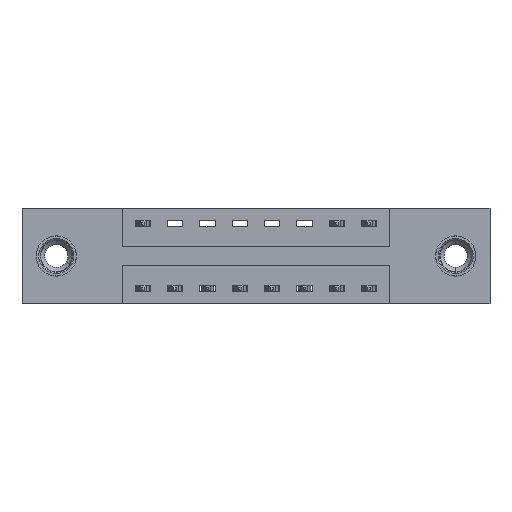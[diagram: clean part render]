
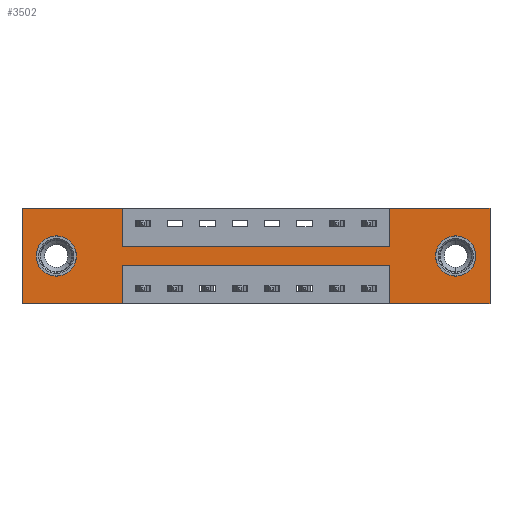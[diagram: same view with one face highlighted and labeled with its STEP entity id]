
A CAD part, front view. The second image highlights one B-rep face of the part: STEP entity #3502.
In plain terms, the highlighted planar face has unit normal (0, -1, 0).
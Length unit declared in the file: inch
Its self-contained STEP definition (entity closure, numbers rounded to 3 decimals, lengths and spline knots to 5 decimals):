
#41 = CARTESIAN_POINT ( 'NONE',  ( 1.6775, 0., -0.185 ) ) ;
#105 = EDGE_CURVE ( 'NONE', #7333, #7266, #4908, .T. ) ;
#182 = LINE ( 'NONE', #8003, #8861 ) ;
#215 = VERTEX_POINT ( 'NONE', #946 ) ;
#295 = LINE ( 'NONE', #981, #8973 ) ;
#345 = DIRECTION ( 'NONE',  ( 0., 0., -1. ) ) ;
#397 = VERTEX_POINT ( 'NONE', #3533 ) ;
#488 = EDGE_CURVE ( 'NONE', #3770, #2480, #9300, .T. ) ;
#666 = VERTEX_POINT ( 'NONE', #4790 ) ;
#691 = LINE ( 'NONE', #5946, #9341 ) ;
#784 = DIRECTION ( 'NONE',  ( -1., 0., 0. ) ) ;
#863 = DIRECTION ( 'NONE',  ( 0., -1., 0. ) ) ;
#910 = DIRECTION ( 'NONE',  ( 0., 0., -1. ) ) ;
#946 = CARTESIAN_POINT ( 'NONE',  ( 0.3875, 0., -0.22 ) ) ;
#981 = CARTESIAN_POINT ( 'NONE',  ( 0., 0., 0. ) ) ;
#1064 = EDGE_CURVE ( 'NONE', #2480, #215, #182, .T. ) ;
#1230 = CARTESIAN_POINT ( 'NONE',  ( 0., 0., -0.37 ) ) ;
#1232 = EDGE_CURVE ( 'NONE', #6895, #3770, #10660, .T. ) ;
#1427 = VERTEX_POINT ( 'NONE', #7745 ) ;
#1442 = EDGE_CURVE ( 'NONE', #7266, #7333, #2202, .T. ) ;
#1566 = AXIS2_PLACEMENT_3D ( 'NONE', #41, #5985, #910 ) ;
#1596 = DIRECTION ( 'NONE',  ( 0., 0., 1. ) ) ;
#1646 = AXIS2_PLACEMENT_3D ( 'NONE', #5944, #863, #6769 ) ;
#1651 = CARTESIAN_POINT ( 'NONE',  ( 1.6775, 0., -0.185 ) ) ;
#1705 = LINE ( 'NONE', #7407, #5918 ) ;
#1753 = CARTESIAN_POINT ( 'NONE',  ( 1.81, 0., 0. ) ) ;
#1877 = FACE_OUTER_BOUND ( 'NONE', #2871, .T. ) ;
#1880 = EDGE_CURVE ( 'NONE', #8380, #397, #1923, .T. ) ;
#1897 = AXIS2_PLACEMENT_3D ( 'NONE', #7795, #7426, #9786 ) ;
#1923 = CIRCLE ( 'NONE', #9036, 0.078 ) ;
#1950 = DIRECTION ( 'NONE',  ( 0., 1., 0. ) ) ;
#2026 = EDGE_CURVE ( 'NONE', #397, #8380, #5330, .T. ) ;
#2086 = EDGE_CURVE ( 'NONE', #1427, #4016, #295, .T. ) ;
#2154 = FACE_BOUND ( 'NONE', #5841, .T. ) ;
#2202 = CIRCLE ( 'NONE', #3690, 0.078 ) ;
#2225 = EDGE_CURVE ( 'NONE', #215, #6181, #7648, .T. ) ;
#2422 = DIRECTION ( 'NONE',  ( -1., 0., 0. ) ) ;
#2480 = VERTEX_POINT ( 'NONE', #8243 ) ;
#2505 = DIRECTION ( 'NONE',  ( 0., 0., -1. ) ) ;
#2755 = CARTESIAN_POINT ( 'NONE',  ( 0.3875, 0., -0.37 ) ) ;
#2871 = EDGE_LOOP ( 'NONE', ( #4343, #4378, #4397, #4405, #4437, #4445, #4464, #4478, #4489, #4503, #4522, #4551 ) ) ;
#2938 = CARTESIAN_POINT ( 'NONE',  ( 0.3875, 0., -0.37 ) ) ;
#3221 = CARTESIAN_POINT ( 'NONE',  ( 1.6775, 0., -0.263 ) ) ;
#3419 = DIRECTION ( 'NONE',  ( 1., 0., 0. ) ) ;
#3502 = ADVANCED_FACE ( 'NONE', ( #4124, #2154, #1877 ), #4250, .T. ) ;
#3510 = EDGE_CURVE ( 'NONE', #4016, #6895, #8283, .T. ) ;
#3533 = CARTESIAN_POINT ( 'NONE',  ( 1.6775, 0., -0.107 ) ) ;
#3690 = AXIS2_PLACEMENT_3D ( 'NONE', #6967, #1950, #7777 ) ;
#3770 = VERTEX_POINT ( 'NONE', #5414 ) ;
#3878 = DIRECTION ( 'NONE',  ( -1., 0., 0. ) ) ;
#4016 = VERTEX_POINT ( 'NONE', #10691 ) ;
#4084 = DIRECTION ( 'NONE',  ( 0., 0., 1. ) ) ;
#4124 = FACE_BOUND ( 'NONE', #7341, .T. ) ;
#4250 = PLANE ( 'NONE',  #1646 ) ;
#4269 = ORIENTED_EDGE ( 'NONE', *, *, #2026, .T. ) ;
#4278 = ORIENTED_EDGE ( 'NONE', *, *, #1880, .T. ) ;
#4301 = ORIENTED_EDGE ( 'NONE', *, *, #1442, .T. ) ;
#4335 = ORIENTED_EDGE ( 'NONE', *, *, #105, .T. ) ;
#4343 = ORIENTED_EDGE ( 'NONE', *, *, #2225, .F. ) ;
#4378 = ORIENTED_EDGE ( 'NONE', *, *, #1064, .F. ) ;
#4397 = ORIENTED_EDGE ( 'NONE', *, *, #488, .F. ) ;
#4402 = DIRECTION ( 'NONE',  ( 0., 0., -1. ) ) ;
#4405 = ORIENTED_EDGE ( 'NONE', *, *, #1232, .F. ) ;
#4437 = ORIENTED_EDGE ( 'NONE', *, *, #3510, .F. ) ;
#4445 = ORIENTED_EDGE ( 'NONE', *, *, #2086, .F. ) ;
#4464 = ORIENTED_EDGE ( 'NONE', *, *, #10239, .F. ) ;
#4478 = ORIENTED_EDGE ( 'NONE', *, *, #8579, .F. ) ;
#4489 = ORIENTED_EDGE ( 'NONE', *, *, #8013, .F. ) ;
#4503 = ORIENTED_EDGE ( 'NONE', *, *, #10445, .F. ) ;
#4522 = ORIENTED_EDGE ( 'NONE', *, *, #9637, .F. ) ;
#4551 = ORIENTED_EDGE ( 'NONE', *, *, #6516, .F. ) ;
#4686 = CARTESIAN_POINT ( 'NONE',  ( 0., 0., 0. ) ) ;
#4790 = CARTESIAN_POINT ( 'NONE',  ( 1.4225, 0., -0.15 ) ) ;
#4801 = LINE ( 'NONE', #9054, #9213 ) ;
#4855 = VECTOR ( 'NONE', #4402, 39.37008 ) ;
#4895 = VECTOR ( 'NONE', #10295, 39.37008 ) ;
#4908 = CIRCLE ( 'NONE', #1897, 0.078 ) ;
#5003 = CARTESIAN_POINT ( 'NONE',  ( 0.1325, 0., -0.107 ) ) ;
#5073 = CARTESIAN_POINT ( 'NONE',  ( 0.1325, 0., -0.263 ) ) ;
#5304 = VERTEX_POINT ( 'NONE', #7276 ) ;
#5330 = CIRCLE ( 'NONE', #1566, 0.078 ) ;
#5342 = CARTESIAN_POINT ( 'NONE',  ( 1.4225, 0., -0.37 ) ) ;
#5372 = CARTESIAN_POINT ( 'NONE',  ( 1.81, 0., -0.37 ) ) ;
#5414 = CARTESIAN_POINT ( 'NONE',  ( 1.4225, 0., -0.37 ) ) ;
#5546 = VERTEX_POINT ( 'NONE', #9369 ) ;
#5841 = EDGE_LOOP ( 'NONE', ( #4301, #4335 ) ) ;
#5902 = CARTESIAN_POINT ( 'NONE',  ( 0.3875, 0., -0.15 ) ) ;
#5918 = VECTOR ( 'NONE', #2422, 39.37008 ) ;
#5944 = CARTESIAN_POINT ( 'NONE',  ( 0., 0., -0.37 ) ) ;
#5946 = CARTESIAN_POINT ( 'NONE',  ( 0., 0., 0. ) ) ;
#5985 = DIRECTION ( 'NONE',  ( 0., 1., 0. ) ) ;
#6181 = VERTEX_POINT ( 'NONE', #2755 ) ;
#6270 = VECTOR ( 'NONE', #784, 39.37008 ) ;
#6349 = VECTOR ( 'NONE', #9224, 39.37008 ) ;
#6361 = VERTEX_POINT ( 'NONE', #4686 ) ;
#6516 = EDGE_CURVE ( 'NONE', #6181, #8176, #1705, .T. ) ;
#6769 = DIRECTION ( 'NONE',  ( 0., 0., -1. ) ) ;
#6879 = DIRECTION ( 'NONE',  ( 1., 0., 0. ) ) ;
#6895 = VERTEX_POINT ( 'NONE', #5372 ) ;
#6967 = CARTESIAN_POINT ( 'NONE',  ( 0.1325, 0., -0.185 ) ) ;
#7266 = VERTEX_POINT ( 'NONE', #5003 ) ;
#7276 = CARTESIAN_POINT ( 'NONE',  ( 0.3875, 0., 0. ) ) ;
#7333 = VERTEX_POINT ( 'NONE', #5073 ) ;
#7341 = EDGE_LOOP ( 'NONE', ( #4269, #4278 ) ) ;
#7407 = CARTESIAN_POINT ( 'NONE',  ( 0., 0., -0.37 ) ) ;
#7426 = DIRECTION ( 'NONE',  ( 0., 1., 0. ) ) ;
#7487 = DIRECTION ( 'NONE',  ( 0., 1., 0. ) ) ;
#7648 = LINE ( 'NONE', #2938, #9616 ) ;
#7698 = CARTESIAN_POINT ( 'NONE',  ( 0.3875, 0., 0. ) ) ;
#7745 = CARTESIAN_POINT ( 'NONE',  ( 1.4225, 0., 0. ) ) ;
#7777 = DIRECTION ( 'NONE',  ( 0., 0., 1. ) ) ;
#7795 = CARTESIAN_POINT ( 'NONE',  ( 0.1325, 0., -0.185 ) ) ;
#8003 = CARTESIAN_POINT ( 'NONE',  ( 0.3875, 0., -0.22 ) ) ;
#8013 = EDGE_CURVE ( 'NONE', #5304, #5546, #9262, .T. ) ;
#8176 = VERTEX_POINT ( 'NONE', #1230 ) ;
#8243 = CARTESIAN_POINT ( 'NONE',  ( 1.4225, 0., -0.22 ) ) ;
#8283 = LINE ( 'NONE', #1753, #6349 ) ;
#8318 = VECTOR ( 'NONE', #1596, 39.37008 ) ;
#8380 = VERTEX_POINT ( 'NONE', #3221 ) ;
#8579 = EDGE_CURVE ( 'NONE', #5546, #666, #8736, .T. ) ;
#8736 = LINE ( 'NONE', #5902, #10671 ) ;
#8861 = VECTOR ( 'NONE', #3878, 39.37008 ) ;
#8973 = VECTOR ( 'NONE', #6879, 39.37008 ) ;
#9036 = AXIS2_PLACEMENT_3D ( 'NONE', #1651, #7487, #2505 ) ;
#9054 = CARTESIAN_POINT ( 'NONE',  ( 1.4225, 0., 0. ) ) ;
#9213 = VECTOR ( 'NONE', #4084, 39.37008 ) ;
#9224 = DIRECTION ( 'NONE',  ( 0., 0., -1. ) ) ;
#9262 = LINE ( 'NONE', #7698, #4855 ) ;
#9300 = LINE ( 'NONE', #5342, #4895 ) ;
#9341 = VECTOR ( 'NONE', #10086, 39.37008 ) ;
#9369 = CARTESIAN_POINT ( 'NONE',  ( 0.3875, 0., -0.15 ) ) ;
#9616 = VECTOR ( 'NONE', #345, 39.37008 ) ;
#9637 = EDGE_CURVE ( 'NONE', #8176, #6361, #10520, .T. ) ;
#9786 = DIRECTION ( 'NONE',  ( 0., 0., 1. ) ) ;
#10086 = DIRECTION ( 'NONE',  ( 1., 0., 0. ) ) ;
#10239 = EDGE_CURVE ( 'NONE', #666, #1427, #4801, .T. ) ;
#10295 = DIRECTION ( 'NONE',  ( 0., 0., 1. ) ) ;
#10445 = EDGE_CURVE ( 'NONE', #6361, #5304, #691, .T. ) ;
#10520 = LINE ( 'NONE', #10754, #8318 ) ;
#10660 = LINE ( 'NONE', #10788, #6270 ) ;
#10671 = VECTOR ( 'NONE', #3419, 39.37008 ) ;
#10691 = CARTESIAN_POINT ( 'NONE',  ( 1.81, 0., 0. ) ) ;
#10754 = CARTESIAN_POINT ( 'NONE',  ( 0., 0., 0. ) ) ;
#10788 = CARTESIAN_POINT ( 'NONE',  ( 0., 0., -0.37 ) ) ;
